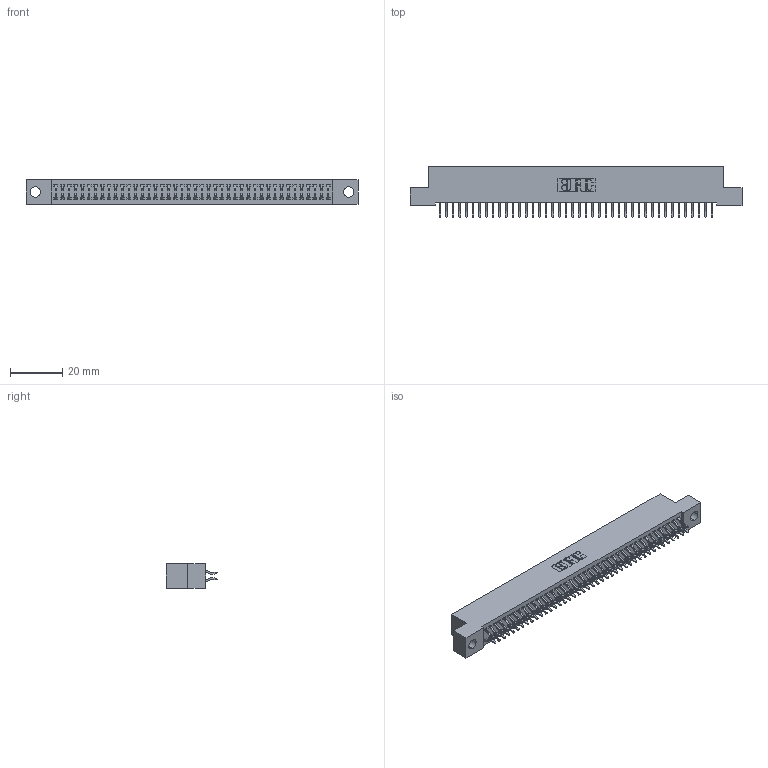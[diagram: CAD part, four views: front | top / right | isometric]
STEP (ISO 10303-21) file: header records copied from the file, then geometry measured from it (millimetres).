
FILE_DESCRIPTION (( 'STEP AP203' ), '1' );
FILE_NAME ('342-084-556-204.STEP', '2019-10-04T12:48:59', ( '' ), ( '' ), 'SwSTEP 2.0', 'SolidWorks 2016', '' );
FILE_SCHEMA (( 'CONFIG_CONTROL_DESIGN' ));
Length unit declared in the file: inch
Products named in the file (3): 345-292-001_556 Tail; 342-084-556-204; 342 Part_.156 TH
Assembly tree (85 placements, depth 2):
  342-084-556-204
    342 Part_.156 TH
    345-292-001_556 Tail  x84
Bounding box: 127 x 19.58 x 9.4 mm (x, y, z)
Volume: 11321.8 mm3; surface area: 18171.7 mm2
Topology: 85 solids, 85 shells, 4982 faces, 14831 edges, 9774 vertices
Faces by surface type: plane 3426, cylinder 1556
Entity records: 27111 total; most frequent: CARTESIAN_POINT 4506, ORIENTED_EDGE 4430, DIRECTION 3839, EDGE_CURVE 2215, LINE 2079, VECTOR 2079, VERTEX_POINT 1474, AXIS2_PLACEMENT_3D 880
